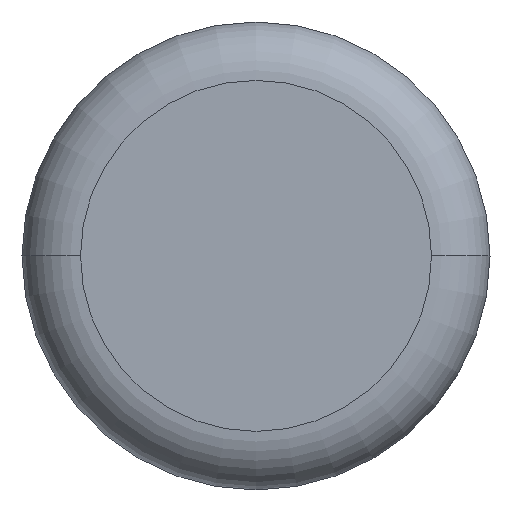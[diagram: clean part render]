
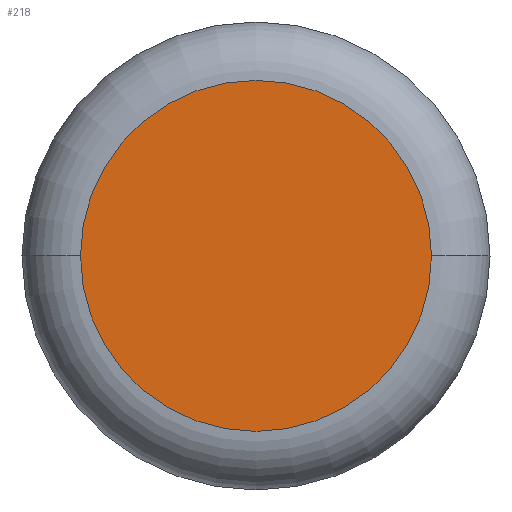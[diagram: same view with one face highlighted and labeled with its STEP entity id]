
A CAD part, top view. The second image highlights one B-rep face of the part: STEP entity #218.
In plain terms, the highlighted planar face has unit normal (0, 0, 1).
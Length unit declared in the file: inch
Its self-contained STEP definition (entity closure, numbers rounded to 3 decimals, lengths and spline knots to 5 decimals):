
#19 = PLANE ( 'NONE',  #227 ) ;
#60 = VERTEX_POINT ( 'NONE', #137 ) ;
#75 = EDGE_CURVE ( 'NONE', #87, #60, #151, .T. ) ;
#82 = CIRCLE ( 'NONE', #216, 0.17717 ) ;
#87 = VERTEX_POINT ( 'NONE', #97 ) ;
#97 = CARTESIAN_POINT ( 'NONE',  ( -0.17717, 0., 1.58268 ) ) ;
#98 = CARTESIAN_POINT ( 'NONE',  ( 0., 0., 1.58268 ) ) ;
#105 = CARTESIAN_POINT ( 'NONE',  ( 0., 0., 1.58268 ) ) ;
#117 = DIRECTION ( 'NONE',  ( 1., 0., 0. ) ) ;
#128 = DIRECTION ( 'NONE',  ( 1., 0., 0. ) ) ;
#137 = CARTESIAN_POINT ( 'NONE',  ( 0.17717, 0., 1.58268 ) ) ;
#151 = CIRCLE ( 'NONE', #256, 0.17717 ) ;
#160 = ORIENTED_EDGE ( 'NONE', *, *, #75, .T. ) ;
#162 = CARTESIAN_POINT ( 'NONE',  ( 0., 0., 1.58268 ) ) ;
#180 = ORIENTED_EDGE ( 'NONE', *, *, #279, .T. ) ;
#181 = DIRECTION ( 'NONE',  ( 0., 0., 1. ) ) ;
#194 = FACE_OUTER_BOUND ( 'NONE', #208, .T. ) ;
#208 = EDGE_LOOP ( 'NONE', ( #180, #160 ) ) ;
#216 = AXIS2_PLACEMENT_3D ( 'NONE', #105, #250, #128 ) ;
#218 = ADVANCED_FACE ( 'NONE', ( #194 ), #19, .T. ) ;
#227 = AXIS2_PLACEMENT_3D ( 'NONE', #162, #181, #261 ) ;
#236 = DIRECTION ( 'NONE',  ( 0., 0., 1. ) ) ;
#250 = DIRECTION ( 'NONE',  ( 0., 0., 1. ) ) ;
#256 = AXIS2_PLACEMENT_3D ( 'NONE', #98, #236, #117 ) ;
#261 = DIRECTION ( 'NONE',  ( 1., 0., 0. ) ) ;
#279 = EDGE_CURVE ( 'NONE', #60, #87, #82, .T. ) ;
